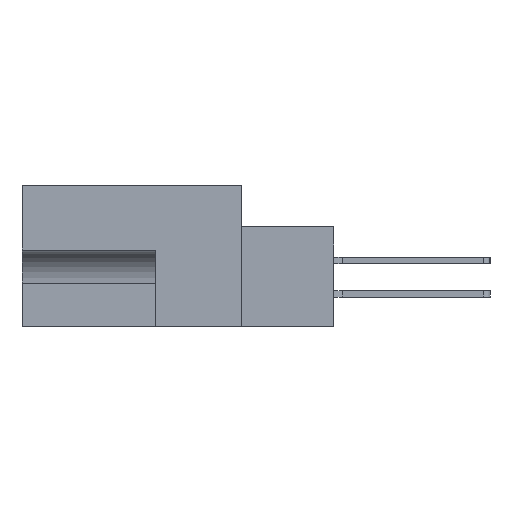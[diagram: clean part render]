
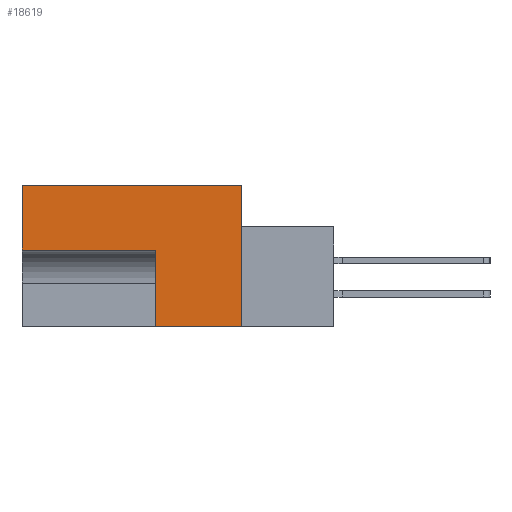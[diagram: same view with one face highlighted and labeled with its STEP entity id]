
A CAD part, left-side view. The second image highlights one B-rep face of the part: STEP entity #18619.
In plain terms, the highlighted planar face has unit normal (-1, 0, 0).
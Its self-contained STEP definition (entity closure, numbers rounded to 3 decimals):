
#965 = ORIENTED_EDGE ( 'NONE', *, *, #18995, .F. ) ;
#2659 = ORIENTED_EDGE ( 'NONE', *, *, #24541, .F. ) ;
#2872 = VERTEX_POINT ( 'NONE', #15463 ) ;
#3394 = CARTESIAN_POINT ( 'NONE',  ( 0., 0., 0. ) ) ;
#3836 = CARTESIAN_POINT ( 'NONE',  ( 0., 0., 0. ) ) ;
#5909 = DIRECTION ( 'NONE',  ( 0., 0., -1. ) ) ;
#6348 = DIRECTION ( 'NONE',  ( 0., 1., 0. ) ) ;
#6733 = LINE ( 'NONE', #24302, #27591 ) ;
#7538 = DIRECTION ( 'NONE',  ( 0., -1., 0. ) ) ;
#8797 = LINE ( 'NONE', #22089, #22397 ) ;
#10300 = ORIENTED_EDGE ( 'NONE', *, *, #24985, .F. ) ;
#10401 = VECTOR ( 'NONE', #6348, 1000. ) ;
#10756 = VERTEX_POINT ( 'NONE', #3836 ) ;
#11081 = EDGE_CURVE ( 'NONE', #12128, #2872, #8797, .T. ) ;
#11844 = FACE_OUTER_BOUND ( 'NONE', #26509, .T. ) ;
#11939 = AXIS2_PLACEMENT_3D ( 'NONE', #3394, #30304, #5909 ) ;
#12128 = VERTEX_POINT ( 'NONE', #29446 ) ;
#13908 = EDGE_CURVE ( 'NONE', #31657, #12128, #24853, .T. ) ;
#13992 = VERTEX_POINT ( 'NONE', #25480 ) ;
#15463 = CARTESIAN_POINT ( 'NONE',  ( 0., 20.955, 0. ) ) ;
#16255 = PLANE ( 'NONE',  #11939 ) ;
#18172 = VECTOR ( 'NONE', #22286, 1000. ) ;
#18619 = ADVANCED_FACE ( 'NONE', ( #11844 ), #16255, .F. ) ;
#18995 = EDGE_CURVE ( 'NONE', #2872, #10756, #6733, .T. ) ;
#19386 = CARTESIAN_POINT ( 'NONE',  ( 0., -8.814, -13.487 ) ) ;
#19878 = LINE ( 'NONE', #22036, #18172 ) ;
#20445 = CARTESIAN_POINT ( 'NONE',  ( 0., 8.255, -6.172 ) ) ;
#21997 = VECTOR ( 'NONE', #23818, 1000. ) ;
#22036 = CARTESIAN_POINT ( 'NONE',  ( 0., 8.255, -13.487 ) ) ;
#22089 = CARTESIAN_POINT ( 'NONE',  ( 0., 20.955, -13.487 ) ) ;
#22112 = DIRECTION ( 'NONE',  ( 0., 1., 0. ) ) ;
#22201 = DIRECTION ( 'NONE',  ( 0., 0., 1. ) ) ;
#22286 = DIRECTION ( 'NONE',  ( 0., 0., 1. ) ) ;
#22397 = VECTOR ( 'NONE', #22201, 1000. ) ;
#23254 = LINE ( 'NONE', #23716, #21997 ) ;
#23716 = CARTESIAN_POINT ( 'NONE',  ( 0., 0., 0. ) ) ;
#23818 = DIRECTION ( 'NONE',  ( 0., 0., -1. ) ) ;
#24302 = CARTESIAN_POINT ( 'NONE',  ( 0., 11.506, 0. ) ) ;
#24441 = VERTEX_POINT ( 'NONE', #29572 ) ;
#24541 = EDGE_CURVE ( 'NONE', #13992, #31657, #19878, .T. ) ;
#24853 = LINE ( 'NONE', #25354, #10401 ) ;
#24985 = EDGE_CURVE ( 'NONE', #24441, #13992, #33042, .T. ) ;
#25354 = CARTESIAN_POINT ( 'NONE',  ( 0., 8.255, -6.172 ) ) ;
#25480 = CARTESIAN_POINT ( 'NONE',  ( 0., 8.255, -13.487 ) ) ;
#25833 = EDGE_CURVE ( 'NONE', #10756, #24441, #23254, .T. ) ;
#26509 = EDGE_LOOP ( 'NONE', ( #10300, #33914, #965, #28921, #28853, #2659 ) ) ;
#27591 = VECTOR ( 'NONE', #7538, 1000. ) ;
#28853 = ORIENTED_EDGE ( 'NONE', *, *, #13908, .F. ) ;
#28921 = ORIENTED_EDGE ( 'NONE', *, *, #11081, .F. ) ;
#29446 = CARTESIAN_POINT ( 'NONE',  ( 0., 20.955, -6.172 ) ) ;
#29572 = CARTESIAN_POINT ( 'NONE',  ( 0., 0., -13.487 ) ) ;
#30304 = DIRECTION ( 'NONE',  ( 1., 0., 0. ) ) ;
#31343 = VECTOR ( 'NONE', #22112, 1000. ) ;
#31657 = VERTEX_POINT ( 'NONE', #20445 ) ;
#33042 = LINE ( 'NONE', #19386, #31343 ) ;
#33914 = ORIENTED_EDGE ( 'NONE', *, *, #25833, .F. ) ;
